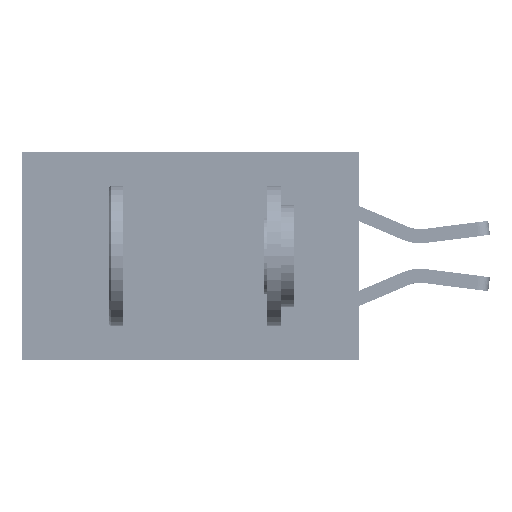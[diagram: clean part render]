
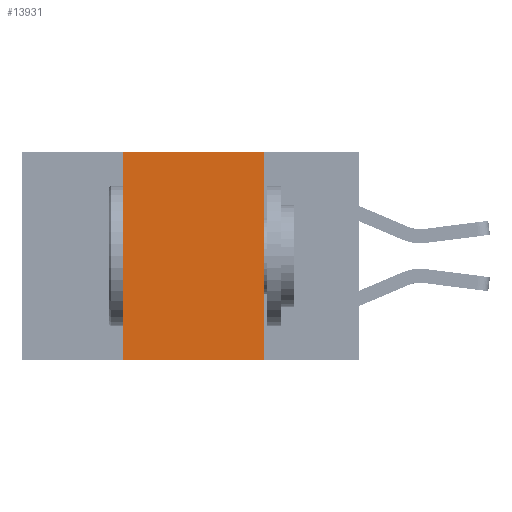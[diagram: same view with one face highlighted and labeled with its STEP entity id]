
A CAD part, left-side view. The second image highlights one B-rep face of the part: STEP entity #13931.
In plain terms, the highlighted planar face has unit normal (-1, 0, 0).
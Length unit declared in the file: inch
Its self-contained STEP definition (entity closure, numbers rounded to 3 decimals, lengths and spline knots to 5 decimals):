
#225 = ORIENTED_EDGE ( 'NONE', *, *, #16109, .F. ) ;
#1677 = CARTESIAN_POINT ( 'NONE',  ( 0., 0.42, -0.37 ) ) ;
#2054 = CARTESIAN_POINT ( 'NONE',  ( 0., 0.42, 0. ) ) ;
#2254 = ORIENTED_EDGE ( 'NONE', *, *, #2520, .F. ) ;
#2520 = EDGE_CURVE ( 'NONE', #21536, #26434, #31574, .T. ) ;
#2639 = VECTOR ( 'NONE', #4802, 39.37008 ) ;
#3486 = ORIENTED_EDGE ( 'NONE', *, *, #18479, .T. ) ;
#3687 = DIRECTION ( 'NONE',  ( 0., -1., 0. ) ) ;
#4802 = DIRECTION ( 'NONE',  ( 0., -1., 0. ) ) ;
#10206 = AXIS2_PLACEMENT_3D ( 'NONE', #20147, #11536, #34653 ) ;
#10764 = DIRECTION ( 'NONE',  ( 0., 0., -1. ) ) ;
#11224 = VECTOR ( 'NONE', #10764, 39.37008 ) ;
#11536 = DIRECTION ( 'NONE',  ( 1., 0., 0. ) ) ;
#13931 = ADVANCED_FACE ( 'NONE', ( #21771 ), #14325, .F. ) ;
#14316 = EDGE_LOOP ( 'NONE', ( #2254, #225, #19321, #3486 ) ) ;
#14325 = PLANE ( 'NONE',  #10206 ) ;
#14782 = EDGE_CURVE ( 'NONE', #17066, #27402, #25787, .T. ) ;
#15909 = CARTESIAN_POINT ( 'NONE',  ( 0., 0.6, -0.37 ) ) ;
#16109 = EDGE_CURVE ( 'NONE', #27402, #21536, #32856, .T. ) ;
#16716 = DIRECTION ( 'NONE',  ( 0., 0., 1. ) ) ;
#17066 = VERTEX_POINT ( 'NONE', #1677 ) ;
#18058 = VECTOR ( 'NONE', #16716, 39.37008 ) ;
#18479 = EDGE_CURVE ( 'NONE', #17066, #26434, #26941, .T. ) ;
#19321 = ORIENTED_EDGE ( 'NONE', *, *, #14782, .F. ) ;
#20147 = CARTESIAN_POINT ( 'NONE',  ( 0., 0.6, 0. ) ) ;
#21061 = VECTOR ( 'NONE', #3687, 39.37008 ) ;
#21536 = VERTEX_POINT ( 'NONE', #36548 ) ;
#21771 = FACE_OUTER_BOUND ( 'NONE', #14316, .T. ) ;
#24163 = CARTESIAN_POINT ( 'NONE',  ( 0., 0.17, -0.37 ) ) ;
#25787 = LINE ( 'NONE', #28255, #18058 ) ;
#26434 = VERTEX_POINT ( 'NONE', #24163 ) ;
#26941 = LINE ( 'NONE', #15909, #21061 ) ;
#27402 = VERTEX_POINT ( 'NONE', #2054 ) ;
#28255 = CARTESIAN_POINT ( 'NONE',  ( 0., 0.42, 0. ) ) ;
#31574 = LINE ( 'NONE', #33888, #11224 ) ;
#32856 = LINE ( 'NONE', #34079, #2639 ) ;
#33888 = CARTESIAN_POINT ( 'NONE',  ( 0., 0.17, 0. ) ) ;
#34079 = CARTESIAN_POINT ( 'NONE',  ( 0., 0.6, 0. ) ) ;
#34653 = DIRECTION ( 'NONE',  ( 0., 0., -1. ) ) ;
#36548 = CARTESIAN_POINT ( 'NONE',  ( 0., 0.17, 0. ) ) ;
